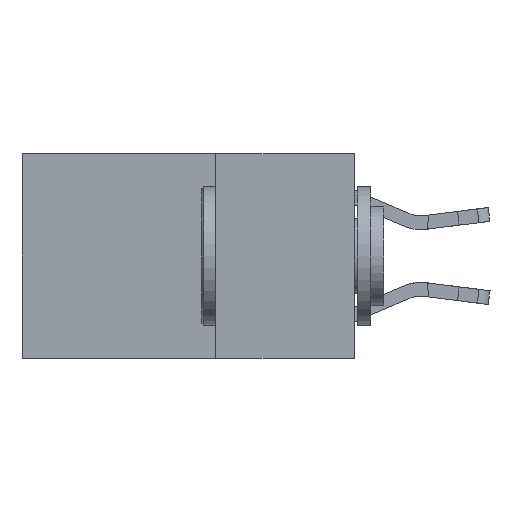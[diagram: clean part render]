
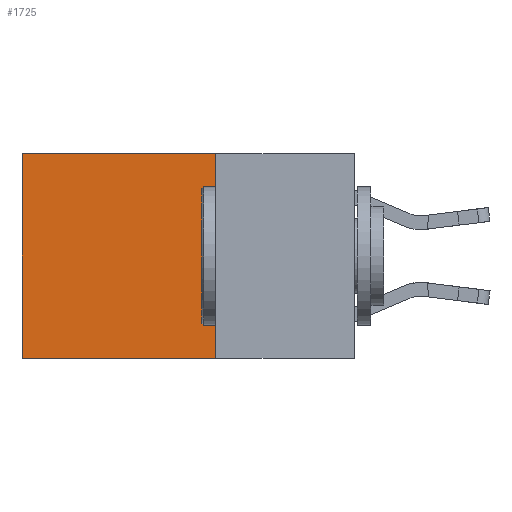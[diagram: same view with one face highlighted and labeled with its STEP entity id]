
A CAD part, left-side view. The second image highlights one B-rep face of the part: STEP entity #1725.
In plain terms, the highlighted planar face has unit normal (-1, 0, 0).
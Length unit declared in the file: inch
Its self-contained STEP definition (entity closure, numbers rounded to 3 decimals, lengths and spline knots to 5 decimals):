
#185 = EDGE_CURVE ( 'NONE', #20363, #18195, #21836, .T. ) ;
#233 = DIRECTION ( 'NONE',  ( 0., 0., -1. ) ) ;
#446 = CARTESIAN_POINT ( 'NONE',  ( 0.2625, 0.6, 0. ) ) ;
#1310 = LINE ( 'NONE', #23478, #18645 ) ;
#1360 = DIRECTION ( 'NONE',  ( 1., 0., 0. ) ) ;
#1725 = ADVANCED_FACE ( 'NONE', ( #9694 ), #12277, .F. ) ;
#1894 = AXIS2_PLACEMENT_3D ( 'NONE', #27141, #1360, #16593 ) ;
#4573 = CARTESIAN_POINT ( 'NONE',  ( 0.2625, 0.25, 0. ) ) ;
#4787 = VECTOR ( 'NONE', #11018, 39.37008 ) ;
#5070 = ORIENTED_EDGE ( 'NONE', *, *, #185, .T. ) ;
#5398 = EDGE_CURVE ( 'NONE', #21544, #12433, #15134, .T. ) ;
#5800 = CARTESIAN_POINT ( 'NONE',  ( 0.2625, 0.25, 0. ) ) ;
#7791 = ORIENTED_EDGE ( 'NONE', *, *, #5398, .F. ) ;
#7924 = EDGE_CURVE ( 'NONE', #21544, #20363, #22665, .T. ) ;
#9694 = FACE_OUTER_BOUND ( 'NONE', #11844, .T. ) ;
#11008 = EDGE_CURVE ( 'NONE', #12433, #18195, #1310, .T. ) ;
#11018 = DIRECTION ( 'NONE',  ( 0., 1., 0. ) ) ;
#11844 = EDGE_LOOP ( 'NONE', ( #5070, #17767, #7791, #12637 ) ) ;
#12277 = PLANE ( 'NONE',  #1894 ) ;
#12433 = VERTEX_POINT ( 'NONE', #13569 ) ;
#12637 = ORIENTED_EDGE ( 'NONE', *, *, #7924, .T. ) ;
#13569 = CARTESIAN_POINT ( 'NONE',  ( 0.2625, 0.25, -0.37 ) ) ;
#15134 = LINE ( 'NONE', #4573, #20141 ) ;
#16207 = VECTOR ( 'NONE', #19984, 39.37008 ) ;
#16593 = DIRECTION ( 'NONE',  ( 0., 0., -1. ) ) ;
#17767 = ORIENTED_EDGE ( 'NONE', *, *, #11008, .F. ) ;
#18097 = CARTESIAN_POINT ( 'NONE',  ( 0.2625, 0.6, -0.37 ) ) ;
#18195 = VERTEX_POINT ( 'NONE', #18097 ) ;
#18645 = VECTOR ( 'NONE', #27716, 39.37008 ) ;
#19984 = DIRECTION ( 'NONE',  ( 0., 0., -1. ) ) ;
#20141 = VECTOR ( 'NONE', #233, 39.37008 ) ;
#20363 = VERTEX_POINT ( 'NONE', #21377 ) ;
#21377 = CARTESIAN_POINT ( 'NONE',  ( 0.2625, 0.6, 0. ) ) ;
#21544 = VERTEX_POINT ( 'NONE', #5800 ) ;
#21657 = CARTESIAN_POINT ( 'NONE',  ( 0.2625, 0.25, 0. ) ) ;
#21836 = LINE ( 'NONE', #446, #16207 ) ;
#22665 = LINE ( 'NONE', #21657, #4787 ) ;
#23478 = CARTESIAN_POINT ( 'NONE',  ( 0.2625, 0.25, -0.37 ) ) ;
#27141 = CARTESIAN_POINT ( 'NONE',  ( 0.2625, 0.25, 0. ) ) ;
#27716 = DIRECTION ( 'NONE',  ( 0., 1., 0. ) ) ;
